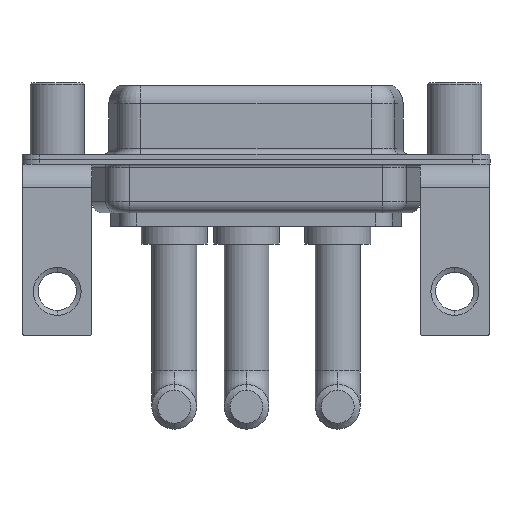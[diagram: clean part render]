
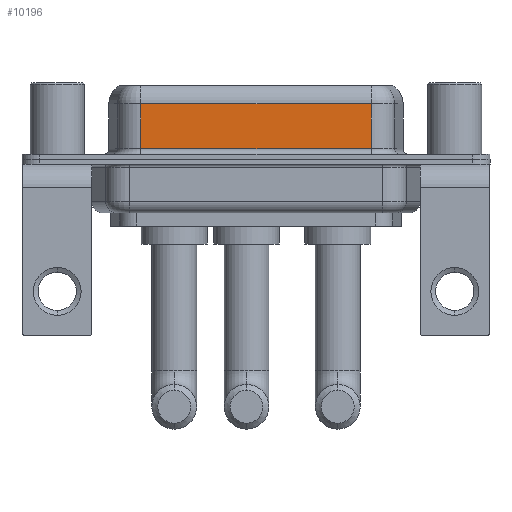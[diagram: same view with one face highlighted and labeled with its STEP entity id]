
A CAD part, front view. The second image highlights one B-rep face of the part: STEP entity #10196.
In plain terms, the highlighted planar face has unit normal (0, -1, 0).
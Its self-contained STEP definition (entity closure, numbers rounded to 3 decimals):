
#32 = CARTESIAN_POINT ( 'NONE',  ( 26.287, -3.95, 4.65 ) ) ;
#78 = ORIENTED_EDGE ( 'NONE', *, *, #11742, .T. ) ;
#405 = EDGE_CURVE ( 'NONE', #11996, #5201, #7873, .T. ) ;
#712 = ORIENTED_EDGE ( 'NONE', *, *, #15166, .F. ) ;
#1190 = DIRECTION ( 'NONE',  ( 0., 1., 0. ) ) ;
#1635 = LINE ( 'NONE', #13825, #8053 ) ;
#3409 = CARTESIAN_POINT ( 'NONE',  ( 26.287, -3.95, 6.4 ) ) ;
#3607 = CARTESIAN_POINT ( 'NONE',  ( 7.013, -3.95, 0.9 ) ) ;
#3817 = DIRECTION ( 'NONE',  ( 0., 0., 1. ) ) ;
#4128 = EDGE_LOOP ( 'NONE', ( #712, #78, #8403, #10834 ) ) ;
#4161 = CARTESIAN_POINT ( 'NONE',  ( 26.287, -3.95, 0.9 ) ) ;
#4810 = VERTEX_POINT ( 'NONE', #32 ) ;
#4894 = AXIS2_PLACEMENT_3D ( 'NONE', #16281, #1190, #3817 ) ;
#5201 = VERTEX_POINT ( 'NONE', #15233 ) ;
#6135 = FACE_OUTER_BOUND ( 'NONE', #4128, .T. ) ;
#6492 = DIRECTION ( 'NONE',  ( 0., 0., -1. ) ) ;
#7873 = LINE ( 'NONE', #4161, #11968 ) ;
#8053 = VECTOR ( 'NONE', #6492, 1000. ) ;
#8403 = ORIENTED_EDGE ( 'NONE', *, *, #10351, .T. ) ;
#9931 = LINE ( 'NONE', #3409, #10036 ) ;
#10036 = VECTOR ( 'NONE', #12315, 1000. ) ;
#10196 = ADVANCED_FACE ( 'NONE', ( #6135 ), #12403, .F. ) ;
#10351 = EDGE_CURVE ( 'NONE', #12115, #11996, #1635, .T. ) ;
#10834 = ORIENTED_EDGE ( 'NONE', *, *, #405, .T. ) ;
#11667 = CARTESIAN_POINT ( 'NONE',  ( 7.013, -3.95, 4.65 ) ) ;
#11742 = EDGE_CURVE ( 'NONE', #4810, #12115, #15011, .T. ) ;
#11968 = VECTOR ( 'NONE', #11986, 1000. ) ;
#11986 = DIRECTION ( 'NONE',  ( 1., 0., 0. ) ) ;
#11996 = VERTEX_POINT ( 'NONE', #3607 ) ;
#12115 = VERTEX_POINT ( 'NONE', #11667 ) ;
#12315 = DIRECTION ( 'NONE',  ( 0., 0., -1. ) ) ;
#12403 = PLANE ( 'NONE',  #4894 ) ;
#12542 = CARTESIAN_POINT ( 'NONE',  ( 26.287, -3.95, 4.65 ) ) ;
#12573 = VECTOR ( 'NONE', #13771, 1000. ) ;
#13771 = DIRECTION ( 'NONE',  ( -1., 0., 0. ) ) ;
#13825 = CARTESIAN_POINT ( 'NONE',  ( 7.013, -3.95, 6.4 ) ) ;
#15011 = LINE ( 'NONE', #12542, #12573 ) ;
#15166 = EDGE_CURVE ( 'NONE', #4810, #5201, #9931, .T. ) ;
#15233 = CARTESIAN_POINT ( 'NONE',  ( 26.287, -3.95, 0.9 ) ) ;
#16281 = CARTESIAN_POINT ( 'NONE',  ( 26.287, -3.95, 6.4 ) ) ;
